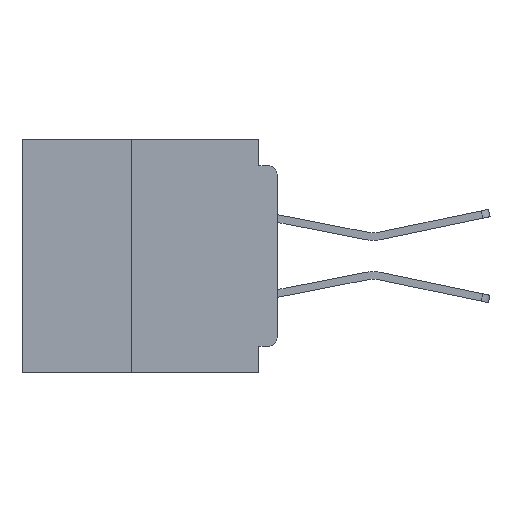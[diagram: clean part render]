
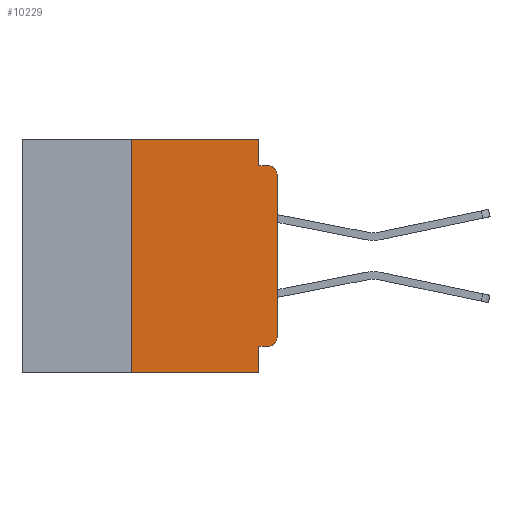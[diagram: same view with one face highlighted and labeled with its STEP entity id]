
A CAD part, left-side view. The second image highlights one B-rep face of the part: STEP entity #10229.
In plain terms, the highlighted planar face has unit normal (-1, 0, 0).
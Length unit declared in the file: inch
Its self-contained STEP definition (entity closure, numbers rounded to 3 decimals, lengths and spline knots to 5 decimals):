
#218 = VECTOR ( 'NONE', #2707, 39.37008 ) ;
#622 = VERTEX_POINT ( 'NONE', #34557 ) ;
#1065 = DIRECTION ( 'NONE',  ( 0., -1., 0. ) ) ;
#2707 = DIRECTION ( 'NONE',  ( 0., 0., 1. ) ) ;
#2897 = VECTOR ( 'NONE', #22135, 39.37008 ) ;
#3507 = CARTESIAN_POINT ( 'NONE',  ( 0., 0.031, -0.4 ) ) ;
#3795 = DIRECTION ( 'NONE',  ( 1., 0., 0. ) ) ;
#3909 = VERTEX_POINT ( 'NONE', #45430 ) ;
#4097 = LINE ( 'NONE', #14453, #2897 ) ;
#4677 = AXIS2_PLACEMENT_3D ( 'NONE', #41733, #3795, #30506 ) ;
#5089 = EDGE_CURVE ( 'NONE', #14807, #33211, #4097, .T. ) ;
#5093 = CARTESIAN_POINT ( 'NONE',  ( 0., 0., 0. ) ) ;
#6554 = CARTESIAN_POINT ( 'NONE',  ( 0., 0.25, -0.4 ) ) ;
#6999 = ORIENTED_EDGE ( 'NONE', *, *, #7035, .T. ) ;
#7035 = EDGE_CURVE ( 'NONE', #10380, #44181, #29536, .T. ) ;
#7130 = ORIENTED_EDGE ( 'NONE', *, *, #9068, .F. ) ;
#8320 = CARTESIAN_POINT ( 'NONE',  ( 0., 0., -0.06 ) ) ;
#9068 = EDGE_CURVE ( 'NONE', #622, #21191, #29807, .T. ) ;
#10219 = ORIENTED_EDGE ( 'NONE', *, *, #40154, .F. ) ;
#10229 = ADVANCED_FACE ( 'NONE', ( #45649 ), #26634, .F. ) ;
#10380 = VERTEX_POINT ( 'NONE', #38939 ) ;
#13884 = EDGE_LOOP ( 'NONE', ( #6999, #28102, #25205, #7130, #10219, #38166, #27889, #48659, #44097, #31864 ) ) ;
#14453 = CARTESIAN_POINT ( 'NONE',  ( 0., 0., -0.355 ) ) ;
#14807 = VERTEX_POINT ( 'NONE', #47934 ) ;
#16584 = DIRECTION ( 'NONE',  ( 0., 0., 1. ) ) ;
#17250 = CARTESIAN_POINT ( 'NONE',  ( 0., 0.437, -0.4 ) ) ;
#18050 = CARTESIAN_POINT ( 'NONE',  ( 0., 0.015, -0.34 ) ) ;
#19105 = CARTESIAN_POINT ( 'NONE',  ( 0., 0.015, -0.045 ) ) ;
#19393 = VECTOR ( 'NONE', #16584, 39.37008 ) ;
#20163 = CARTESIAN_POINT ( 'NONE',  ( 0., 0.015, -0.06 ) ) ;
#21116 = DIRECTION ( 'NONE',  ( 0., -1., 0. ) ) ;
#21191 = VERTEX_POINT ( 'NONE', #44696 ) ;
#21902 = DIRECTION ( 'NONE',  ( 0., 0., -1. ) ) ;
#21925 = LINE ( 'NONE', #49043, #40898 ) ;
#22135 = DIRECTION ( 'NONE',  ( 0., 1., 0. ) ) ;
#23329 = EDGE_CURVE ( 'NONE', #3909, #32518, #30384, .T. ) ;
#23942 = DIRECTION ( 'NONE',  ( 0., 0., -1. ) ) ;
#24037 = EDGE_CURVE ( 'NONE', #33211, #32518, #28521, .T. ) ;
#25205 = ORIENTED_EDGE ( 'NONE', *, *, #48042, .F. ) ;
#26098 = VECTOR ( 'NONE', #34028, 39.37008 ) ;
#26107 = EDGE_CURVE ( 'NONE', #14807, #10380, #35442, .T. ) ;
#26420 = DIRECTION ( 'NONE',  ( 0., -1., 0. ) ) ;
#26634 = PLANE ( 'NONE',  #4677 ) ;
#27432 = VECTOR ( 'NONE', #37219, 39.37008 ) ;
#27889 = ORIENTED_EDGE ( 'NONE', *, *, #23329, .T. ) ;
#28102 = ORIENTED_EDGE ( 'NONE', *, *, #46096, .T. ) ;
#28521 = LINE ( 'NONE', #3507, #26098 ) ;
#29206 = AXIS2_PLACEMENT_3D ( 'NONE', #18050, #44614, #21902 ) ;
#29536 = LINE ( 'NONE', #5093, #19393 ) ;
#29807 = LINE ( 'NONE', #48371, #27432 ) ;
#30384 = LINE ( 'NONE', #17250, #49232 ) ;
#30506 = DIRECTION ( 'NONE',  ( 0., 0., -1. ) ) ;
#31864 = ORIENTED_EDGE ( 'NONE', *, *, #26107, .T. ) ;
#32518 = VERTEX_POINT ( 'NONE', #41214 ) ;
#33211 = VERTEX_POINT ( 'NONE', #35179 ) ;
#33703 = VECTOR ( 'NONE', #1065, 39.37008 ) ;
#34028 = DIRECTION ( 'NONE',  ( 0., 0., -1. ) ) ;
#34557 = CARTESIAN_POINT ( 'NONE',  ( 0., 0.031, 0. ) ) ;
#35179 = CARTESIAN_POINT ( 'NONE',  ( 0., 0.031, -0.355 ) ) ;
#35442 = CIRCLE ( 'NONE', #29206, 0.015 ) ;
#37219 = DIRECTION ( 'NONE',  ( 0., 0., -1. ) ) ;
#38150 = VERTEX_POINT ( 'NONE', #40186 ) ;
#38166 = ORIENTED_EDGE ( 'NONE', *, *, #40435, .F. ) ;
#38473 = AXIS2_PLACEMENT_3D ( 'NONE', #20163, #46644, #23942 ) ;
#38939 = CARTESIAN_POINT ( 'NONE',  ( 0., 0., -0.34 ) ) ;
#40006 = VERTEX_POINT ( 'NONE', #19105 ) ;
#40154 = EDGE_CURVE ( 'NONE', #38150, #622, #44241, .T. ) ;
#40186 = CARTESIAN_POINT ( 'NONE',  ( 0., 0.25, 0. ) ) ;
#40435 = EDGE_CURVE ( 'NONE', #3909, #38150, #40730, .T. ) ;
#40730 = LINE ( 'NONE', #6554, #218 ) ;
#40898 = VECTOR ( 'NONE', #26420, 39.37008 ) ;
#41034 = CIRCLE ( 'NONE', #38473, 0.015 ) ;
#41214 = CARTESIAN_POINT ( 'NONE',  ( 0., 0.031, -0.4 ) ) ;
#41733 = CARTESIAN_POINT ( 'NONE',  ( 0., 0.437, 0. ) ) ;
#44097 = ORIENTED_EDGE ( 'NONE', *, *, #5089, .F. ) ;
#44181 = VERTEX_POINT ( 'NONE', #8320 ) ;
#44241 = LINE ( 'NONE', #46591, #33703 ) ;
#44614 = DIRECTION ( 'NONE',  ( -1., 0., 0. ) ) ;
#44696 = CARTESIAN_POINT ( 'NONE',  ( 0., 0.031, -0.045 ) ) ;
#45430 = CARTESIAN_POINT ( 'NONE',  ( 0., 0.25, -0.4 ) ) ;
#45649 = FACE_OUTER_BOUND ( 'NONE', #13884, .T. ) ;
#46096 = EDGE_CURVE ( 'NONE', #44181, #40006, #41034, .T. ) ;
#46591 = CARTESIAN_POINT ( 'NONE',  ( 0., 0.437, 0. ) ) ;
#46644 = DIRECTION ( 'NONE',  ( -1., 0., 0. ) ) ;
#47934 = CARTESIAN_POINT ( 'NONE',  ( 0., 0.015, -0.355 ) ) ;
#48042 = EDGE_CURVE ( 'NONE', #21191, #40006, #21925, .T. ) ;
#48371 = CARTESIAN_POINT ( 'NONE',  ( 0., 0.031, 0. ) ) ;
#48659 = ORIENTED_EDGE ( 'NONE', *, *, #24037, .F. ) ;
#49043 = CARTESIAN_POINT ( 'NONE',  ( 0., 0., -0.045 ) ) ;
#49232 = VECTOR ( 'NONE', #21116, 39.37008 ) ;
